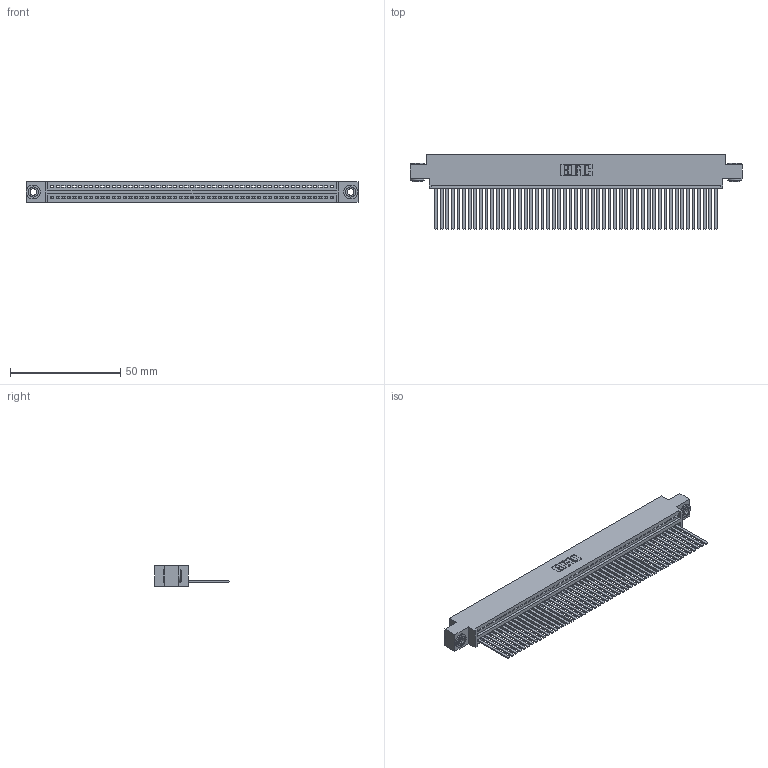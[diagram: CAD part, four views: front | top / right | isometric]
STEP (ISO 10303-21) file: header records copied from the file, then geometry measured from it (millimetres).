
FILE_DESCRIPTION (( 'STEP AP203' ), '1' );
FILE_NAME ('345-051-544-603.STEP', '2019-10-09T16:43:12', ( '' ), ( '' ), 'SwSTEP 2.0', 'SolidWorks 2016', '' );
FILE_SCHEMA (( 'CONFIG_CONTROL_DESIGN' ));
Length unit declared in the file: inch
Products named in the file (4): 345 Part_0.170 Offset - 0.156 Dia-TH; 345-292-001_345-293-144; 345-051-544-603; 345-250-002_345-250-002-102
Assembly tree (54 placements, depth 2):
  345-051-544-603
    345 Part_0.170 Offset - 0.156 Dia-TH
    345-292-001_345-293-144  x51
    345-250-002_345-250-002-102  x2
Bounding box: 150.75 x 33.96 x 9.4 mm (x, y, z)
Volume: 14888.7 mm3; surface area: 22022.2 mm2
Topology: 54 solids, 54 shells, 2820 faces, 8487 edges, 5586 vertices
Faces by surface type: plane 1930, cylinder 882, cone 8
Entity records: 37770 total; most frequent: CARTESIAN_POINT 6520, ORIENTED_EDGE 6498, DIRECTION 5709, EDGE_CURVE 3249, LINE 2893, VECTOR 2893, VERTEX_POINT 2162, AXIS2_PLACEMENT_3D 1408
